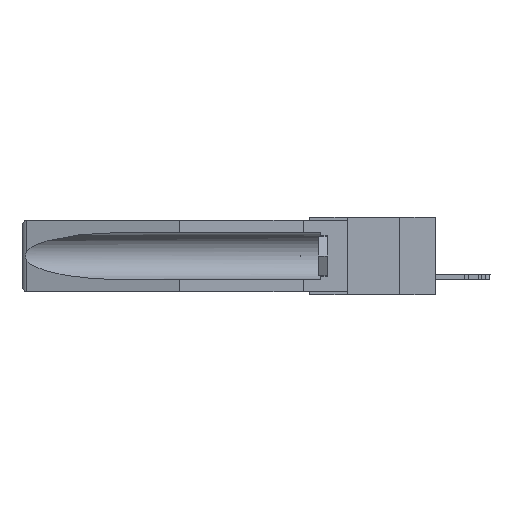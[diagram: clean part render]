
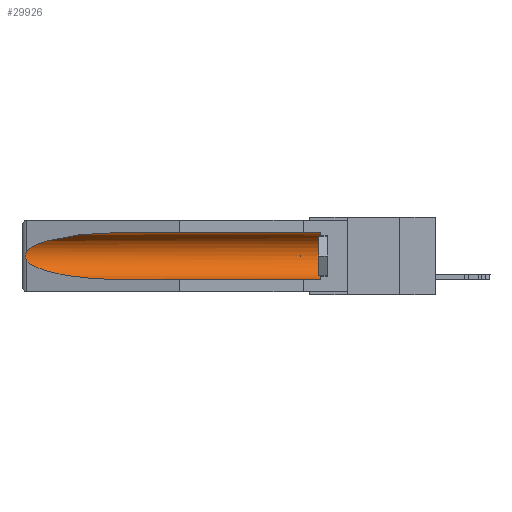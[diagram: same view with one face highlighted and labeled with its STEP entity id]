
A CAD part, left-side view. The second image highlights one B-rep face of the part: STEP entity #29926.
In plain terms, the highlighted cylindrical face has radius 2.857 mm (diameter 5.715 mm), a partial arc.
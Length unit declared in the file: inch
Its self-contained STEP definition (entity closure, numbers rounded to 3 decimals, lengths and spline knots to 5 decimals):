
#44 = CARTESIAN_POINT ( 'NONE',  ( 0.155, 1.07973, -0.284 ) ) ;
#1134 = VERTEX_POINT ( 'NONE', #44 ) ;
#1323 = CARTESIAN_POINT ( 'NONE',  ( 0.26597, 1.5296, -0.19026 ) ) ;
#1356 = EDGE_CURVE ( 'NONE', #21287, #21429, #4374, .T. ) ;
#1578 = DIRECTION ( 'NONE',  ( 0., -1., 0. ) ) ;
#1669 = CARTESIAN_POINT ( 'NONE',  ( 0.26597, 1.52961, -0.15275 ) ) ;
#1693 = DIRECTION ( 'NONE',  ( 0., 1., 0. ) ) ;
#3052 = DIRECTION ( 'NONE',  ( 0., 1., 0. ) ) ;
#3443 = EDGE_CURVE ( 'NONE', #21429, #31186, #25800, .T. ) ;
#3830 = CARTESIAN_POINT ( 'NONE',  ( 0.155, -0.30754, -0.1715 ) ) ;
#3935 = DIRECTION ( 'NONE',  ( 0., 0., 1. ) ) ;
#4132 = CARTESIAN_POINT ( 'NONE',  ( 0.26537, 1.52718, -0.19328 ) ) ;
#4374 = CIRCLE ( 'NONE', #6318, 0.1125 ) ;
#6318 = AXIS2_PLACEMENT_3D ( 'NONE', #22525, #1578, #27770 ) ;
#6659 = CARTESIAN_POINT ( 'NONE',  ( 0.2675, 1.53308, -0.17534 ) ) ;
#7159 = ORIENTED_EDGE ( 'NONE', *, *, #7191, .T. ) ;
#7191 = EDGE_CURVE ( 'NONE', #28308, #1134, #31923, .T. ) ;
#7449 = CARTESIAN_POINT ( 'NONE',  ( 0.25451, 1.48313, -0.24835 ) ) ;
#7464 = VECTOR ( 'NONE', #19490, 39.37008 ) ;
#7557 = CARTESIAN_POINT ( 'NONE',  ( 0.26537, 1.52718, -0.14972 ) ) ;
#7591 = CARTESIAN_POINT ( 'NONE',  ( 0.155, 0.126, -0.284 ) ) ;
#8885 = CARTESIAN_POINT ( 'NONE',  ( 0.26537, 1.52718, -0.19328 ) ) ;
#9151 = CARTESIAN_POINT ( 'NONE',  ( 0.26654, 1.53092, -0.15636 ) ) ;
#9757 = B_SPLINE_CURVE_WITH_KNOTS ( 'NONE', 3,
 ( #32865, #1669, #9151, #27157, #25004, #6659, #19396, #32638, #1323, #27394 ),
 .UNSPECIFIED., .F., .F.,
 ( 4, 2, 2, 2, 4 ),
 ( 0., 0.00029, 0.00058, 0.00087, 0.00117 ),
 .UNSPECIFIED. ) ;
#10695 = CARTESIAN_POINT ( 'NONE',  ( 0.155, 1.07973, -0.059 ) ) ;
#12740 = CYLINDRICAL_SURFACE ( 'NONE', #26792, 0.1125 ) ;
#13240 = VECTOR ( 'NONE', #3052, 39.37008 ) ;
#13957 = FACE_OUTER_BOUND ( 'NONE', #28745, .T. ) ;
#14283 = ORIENTED_EDGE ( 'NONE', *, *, #22715, .F. ) ;
#14806 = ORIENTED_EDGE ( 'NONE', *, *, #3443, .T. ) ;
#14825 = EDGE_CURVE ( 'NONE', #31186, #20302, #27934, .T. ) ;
#15898 = ORIENTED_EDGE ( 'NONE', *, *, #1356, .T. ) ;
#16703 = EDGE_CURVE ( 'NONE', #20302, #28308, #9757, .T. ) ;
#18455 = ORIENTED_EDGE ( 'NONE', *, *, #16703, .T. ) ;
#19396 = CARTESIAN_POINT ( 'NONE',  ( 0.2673, 1.53269, -0.17917 ) ) ;
#19490 = DIRECTION ( 'NONE',  ( 0., 1., 0. ) ) ;
#20144 = LINE ( 'NONE', #24032, #13240 ) ;
#20302 = VERTEX_POINT ( 'NONE', #7557 ) ;
#21287 = VERTEX_POINT ( 'NONE', #7591 ) ;
#21429 = VERTEX_POINT ( 'NONE', #21699 ) ;
#21699 = CARTESIAN_POINT ( 'NONE',  ( 0.155, 0.126, -0.059 ) ) ;
#21939 = ORIENTED_EDGE ( 'NONE', *, *, #14825, .T. ) ;
#22061 = CARTESIAN_POINT ( 'NONE',  ( 0.26537, 1.52718, -0.14972 ) ) ;
#22344 = CARTESIAN_POINT ( 'NONE',  ( 0.155, -0.30754, -0.059 ) ) ;
#22525 = CARTESIAN_POINT ( 'NONE',  ( 0.155, 0.126, -0.1715 ) ) ;
#22715 = EDGE_CURVE ( 'NONE', #21287, #1134, #20144, .T. ) ;
#24032 = CARTESIAN_POINT ( 'NONE',  ( 0.155, -0.30754, -0.284 ) ) ;
#24809 = CARTESIAN_POINT ( 'NONE',  ( 0.21114, 1.30732, -0.059 ) ) ;
#25004 = CARTESIAN_POINT ( 'NONE',  ( 0.2675, 1.53308, -0.16763 ) ) ;
#25103 = CARTESIAN_POINT ( 'NONE',  ( 0.21114, 1.30732, -0.284 ) ) ;
#25677 = CARTESIAN_POINT ( 'NONE',  ( 0.155, 1.07973, -0.284 ) ) ;
#25800 = LINE ( 'NONE', #22344, #7464 ) ;
#26792 = AXIS2_PLACEMENT_3D ( 'NONE', #3830, #1693, #3935 ) ;
#27157 = CARTESIAN_POINT ( 'NONE',  ( 0.2673, 1.5327, -0.16383 ) ) ;
#27394 = CARTESIAN_POINT ( 'NONE',  ( 0.26537, 1.52718, -0.19328 ) ) ;
#27541 = CARTESIAN_POINT ( 'NONE',  ( 0.25451, 1.48313, -0.09465 ) ) ;
#27770 = DIRECTION ( 'NONE',  ( 0., 0., 1. ) ) ;
#27934 =( BOUNDED_CURVE ( )  B_SPLINE_CURVE ( 3, ( #29914, #24809, #27541, #22061 ),
 .UNSPECIFIED., .F., .T. ) 
 B_SPLINE_CURVE_WITH_KNOTS ( ( 4, 4 ),
 ( 4.71239, 6.08839 ),
 .UNSPECIFIED. ) 
 CURVE ( )  GEOMETRIC_REPRESENTATION_ITEM ( )  RATIONAL_B_SPLINE_CURVE ( ( 1., 0.848, 0.848, 1. ) ) 
 REPRESENTATION_ITEM ( '' )  );
#28308 = VERTEX_POINT ( 'NONE', #8885 ) ;
#28745 = EDGE_LOOP ( 'NONE', ( #21939, #18455, #7159, #14283, #15898, #14806 ) ) ;
#29914 = CARTESIAN_POINT ( 'NONE',  ( 0.155, 1.07973, -0.059 ) ) ;
#29926 = ADVANCED_FACE ( 'NONE', ( #13957 ), #12740, .F. ) ;
#31186 = VERTEX_POINT ( 'NONE', #10695 ) ;
#31923 =( BOUNDED_CURVE ( )  B_SPLINE_CURVE ( 3, ( #4132, #7449, #25103, #25677 ),
 .UNSPECIFIED., .F., .T. ) 
 B_SPLINE_CURVE_WITH_KNOTS ( ( 4, 4 ),
 ( 0.1948, 1.5708 ),
 .UNSPECIFIED. ) 
 CURVE ( )  GEOMETRIC_REPRESENTATION_ITEM ( )  RATIONAL_B_SPLINE_CURVE ( ( 1., 0.848, 0.848, 1. ) ) 
 REPRESENTATION_ITEM ( '' )  );
#32638 = CARTESIAN_POINT ( 'NONE',  ( 0.26655, 1.53094, -0.18657 ) ) ;
#32865 = CARTESIAN_POINT ( 'NONE',  ( 0.26537, 1.52718, -0.14972 ) ) ;
